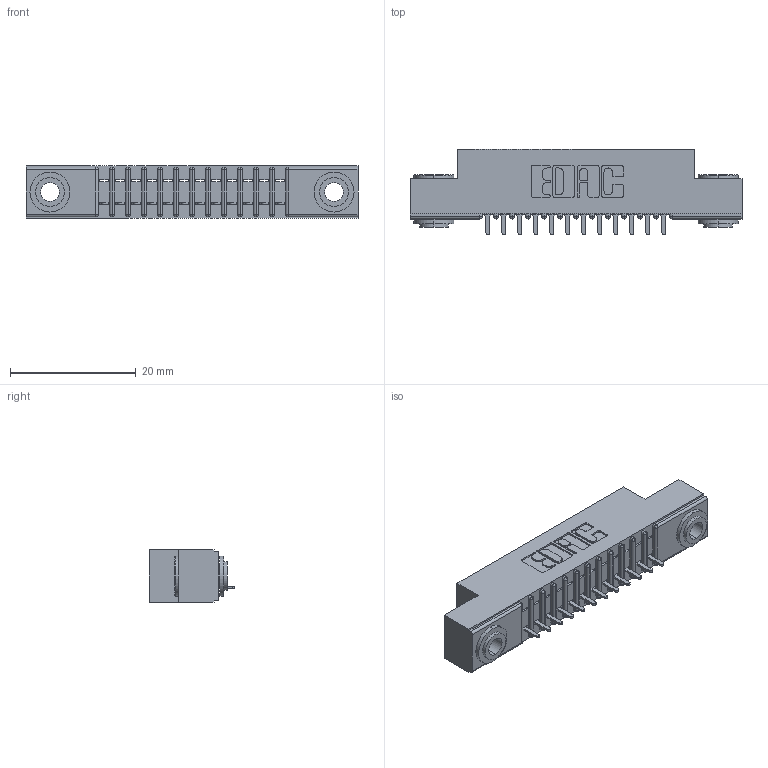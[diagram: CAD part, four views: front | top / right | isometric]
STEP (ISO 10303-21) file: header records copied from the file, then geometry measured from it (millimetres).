
FILE_DESCRIPTION (( 'STEP AP203' ), '1' );
FILE_NAME ('391-012-524-103.STEP', '2018-08-08T16:35:03', ( '' ), ( '' ), 'SwSTEP 2.0', 'SolidWorks 2016', '' );
FILE_SCHEMA (( 'CONFIG_CONTROL_DESIGN' ));
Length unit declared in the file: inch
Products named in the file (4): 341-292-001_341-292-124; 345-250-002_345-250-002-102; 391-012-524-103; 341 Part_.156 (3.96) Dia Mounting Holes
Assembly tree (15 placements, depth 2):
  391-012-524-103
    341 Part_.156 (3.96) Dia Mounting Holes
    341-292-001_341-292-124  x12
    345-250-002_345-250-002-102  x2
Bounding box: 52.7 x 13.64 x 8.38 mm (x, y, z)
Volume: 2942.1 mm3; surface area: 5162.1 mm2
Topology: 15 solids, 15 shells, 1152 faces, 3272 edges, 2102 vertices
Faces by surface type: plane 704, cylinder 392, sphere 26, torus 22, cone 8
Entity records: 19200 total; most frequent: CARTESIAN_POINT 3225, ORIENTED_EDGE 3204, DIRECTION 3154, EDGE_CURVE 1602, LINE 1252, VECTOR 1252, VERTEX_POINT 1022, AXIS2_PLACEMENT_3D 951
